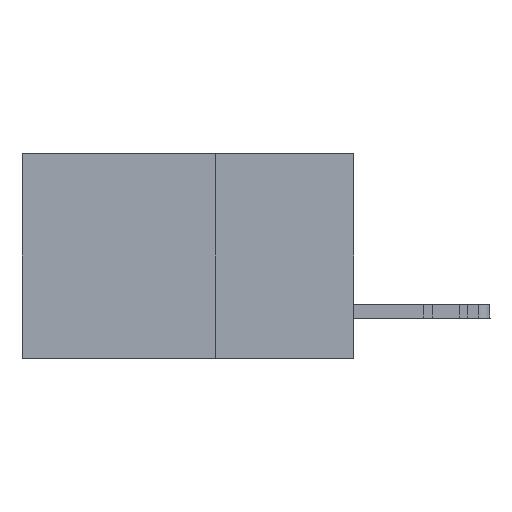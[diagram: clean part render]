
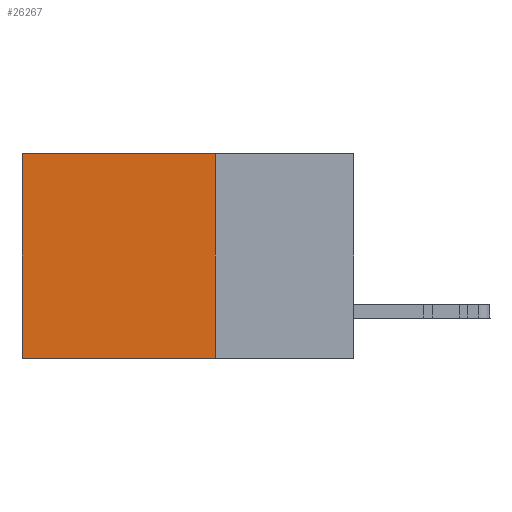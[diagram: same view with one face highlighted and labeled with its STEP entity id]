
A CAD part, left-side view. The second image highlights one B-rep face of the part: STEP entity #26267.
In plain terms, the highlighted planar face has unit normal (-1, 0, 0).
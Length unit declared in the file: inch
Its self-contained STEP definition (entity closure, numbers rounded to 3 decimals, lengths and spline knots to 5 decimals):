
#2091 = VERTEX_POINT ( 'NONE', #32051 ) ;
#2792 = DIRECTION ( 'NONE',  ( 1., 0., 0. ) ) ;
#2796 = CARTESIAN_POINT ( 'NONE',  ( 0.2875, 0.25, 0. ) ) ;
#3676 = VERTEX_POINT ( 'NONE', #2796 ) ;
#7746 = LINE ( 'NONE', #20328, #31491 ) ;
#9487 = DIRECTION ( 'NONE',  ( 0., 0., -1. ) ) ;
#9730 = CARTESIAN_POINT ( 'NONE',  ( 0.2875, 0.25, 0. ) ) ;
#12275 = CARTESIAN_POINT ( 'NONE',  ( 0.2875, 0.6, 0. ) ) ;
#12422 = DIRECTION ( 'NONE',  ( 0., 0., -1. ) ) ;
#13456 = VERTEX_POINT ( 'NONE', #24502 ) ;
#14656 = FACE_OUTER_BOUND ( 'NONE', #35661, .T. ) ;
#16827 = ORIENTED_EDGE ( 'NONE', *, *, #23143, .T. ) ;
#18802 = ORIENTED_EDGE ( 'NONE', *, *, #44637, .T. ) ;
#19386 = CARTESIAN_POINT ( 'NONE',  ( 0.2875, 0.6, 0. ) ) ;
#20328 = CARTESIAN_POINT ( 'NONE',  ( 0.2875, 0.25, 0. ) ) ;
#20624 = VECTOR ( 'NONE', #22800, 39.37008 ) ;
#22800 = DIRECTION ( 'NONE',  ( 0., 1., 0. ) ) ;
#23143 = EDGE_CURVE ( 'NONE', #3676, #25567, #7746, .T. ) ;
#23901 = DIRECTION ( 'NONE',  ( 0., 1., 0. ) ) ;
#24502 = CARTESIAN_POINT ( 'NONE',  ( 0.2875, 0.25, -0.37 ) ) ;
#25567 = VERTEX_POINT ( 'NONE', #12275 ) ;
#26159 = LINE ( 'NONE', #19386, #28919 ) ;
#26164 = AXIS2_PLACEMENT_3D ( 'NONE', #9730, #2792, #34394 ) ;
#26267 = ADVANCED_FACE ( 'NONE', ( #14656 ), #30872, .F. ) ;
#28609 = VECTOR ( 'NONE', #9487, 39.37008 ) ;
#28919 = VECTOR ( 'NONE', #12422, 39.37008 ) ;
#30872 = PLANE ( 'NONE',  #26164 ) ;
#31401 = EDGE_CURVE ( 'NONE', #13456, #2091, #42729, .T. ) ;
#31491 = VECTOR ( 'NONE', #23901, 39.37008 ) ;
#32051 = CARTESIAN_POINT ( 'NONE',  ( 0.2875, 0.6, -0.37 ) ) ;
#33997 = CARTESIAN_POINT ( 'NONE',  ( 0.2875, 0.25, 0. ) ) ;
#34059 = ORIENTED_EDGE ( 'NONE', *, *, #34614, .F. ) ;
#34394 = DIRECTION ( 'NONE',  ( 0., 0., -1. ) ) ;
#34614 = EDGE_CURVE ( 'NONE', #3676, #13456, #44046, .T. ) ;
#35661 = EDGE_LOOP ( 'NONE', ( #18802, #40460, #34059, #16827 ) ) ;
#37290 = CARTESIAN_POINT ( 'NONE',  ( 0.2875, 0.25, -0.37 ) ) ;
#40460 = ORIENTED_EDGE ( 'NONE', *, *, #31401, .F. ) ;
#42729 = LINE ( 'NONE', #37290, #20624 ) ;
#44046 = LINE ( 'NONE', #33997, #28609 ) ;
#44637 = EDGE_CURVE ( 'NONE', #25567, #2091, #26159, .T. ) ;
